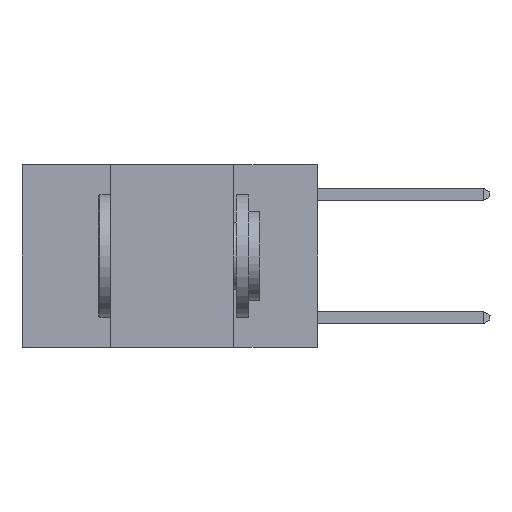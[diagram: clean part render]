
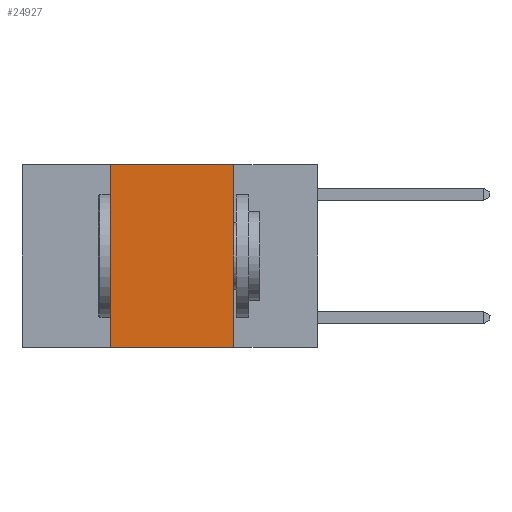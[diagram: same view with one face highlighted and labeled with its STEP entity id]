
A CAD part, left-side view. The second image highlights one B-rep face of the part: STEP entity #24927.
In plain terms, the highlighted planar face has unit normal (-1, 0, 0).
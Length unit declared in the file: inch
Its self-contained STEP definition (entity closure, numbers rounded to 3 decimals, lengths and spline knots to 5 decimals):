
#614 = VECTOR ( 'NONE', #22549, 39.37008 ) ;
#1369 = DIRECTION ( 'NONE',  ( 0., 0., -1. ) ) ;
#1462 = VERTEX_POINT ( 'NONE', #3808 ) ;
#2837 = LINE ( 'NONE', #16301, #25153 ) ;
#3808 = CARTESIAN_POINT ( 'NONE',  ( 0., 0.17, -0.37 ) ) ;
#6460 = LINE ( 'NONE', #20490, #614 ) ;
#9163 = DIRECTION ( 'NONE',  ( 0., 0., -1. ) ) ;
#9464 = AXIS2_PLACEMENT_3D ( 'NONE', #19521, #21560, #9163 ) ;
#11378 = LINE ( 'NONE', #20600, #21718 ) ;
#11495 = ORIENTED_EDGE ( 'NONE', *, *, #25972, .T. ) ;
#13531 = VERTEX_POINT ( 'NONE', #26478 ) ;
#14460 = EDGE_LOOP ( 'NONE', ( #15083, #21194, #26647, #11495 ) ) ;
#14592 = EDGE_CURVE ( 'NONE', #13531, #15224, #19726, .T. ) ;
#15083 = ORIENTED_EDGE ( 'NONE', *, *, #21834, .F. ) ;
#15224 = VERTEX_POINT ( 'NONE', #15950 ) ;
#15905 = VERTEX_POINT ( 'NONE', #16373 ) ;
#15950 = CARTESIAN_POINT ( 'NONE',  ( 0., 0.17, 0. ) ) ;
#15984 = CARTESIAN_POINT ( 'NONE',  ( 0., 0.6, 0. ) ) ;
#16301 = CARTESIAN_POINT ( 'NONE',  ( 0., 0.17, 0. ) ) ;
#16373 = CARTESIAN_POINT ( 'NONE',  ( 0., 0.42, -0.37 ) ) ;
#17427 = PLANE ( 'NONE',  #9464 ) ;
#18432 = VECTOR ( 'NONE', #22179, 39.37008 ) ;
#19521 = CARTESIAN_POINT ( 'NONE',  ( 0., 0.6, 0. ) ) ;
#19726 = LINE ( 'NONE', #15984, #18432 ) ;
#20490 = CARTESIAN_POINT ( 'NONE',  ( 0., 0.42, 0. ) ) ;
#20600 = CARTESIAN_POINT ( 'NONE',  ( 0., 0.6, -0.37 ) ) ;
#21194 = ORIENTED_EDGE ( 'NONE', *, *, #14592, .F. ) ;
#21560 = DIRECTION ( 'NONE',  ( 1., 0., 0. ) ) ;
#21718 = VECTOR ( 'NONE', #24751, 39.37008 ) ;
#21834 = EDGE_CURVE ( 'NONE', #15224, #1462, #2837, .T. ) ;
#22179 = DIRECTION ( 'NONE',  ( 0., -1., 0. ) ) ;
#22549 = DIRECTION ( 'NONE',  ( 0., 0., 1. ) ) ;
#24593 = EDGE_CURVE ( 'NONE', #15905, #13531, #6460, .T. ) ;
#24751 = DIRECTION ( 'NONE',  ( 0., -1., 0. ) ) ;
#24927 = ADVANCED_FACE ( 'NONE', ( #26271 ), #17427, .F. ) ;
#25153 = VECTOR ( 'NONE', #1369, 39.37008 ) ;
#25972 = EDGE_CURVE ( 'NONE', #15905, #1462, #11378, .T. ) ;
#26271 = FACE_OUTER_BOUND ( 'NONE', #14460, .T. ) ;
#26478 = CARTESIAN_POINT ( 'NONE',  ( 0., 0.42, 0. ) ) ;
#26647 = ORIENTED_EDGE ( 'NONE', *, *, #24593, .F. ) ;
